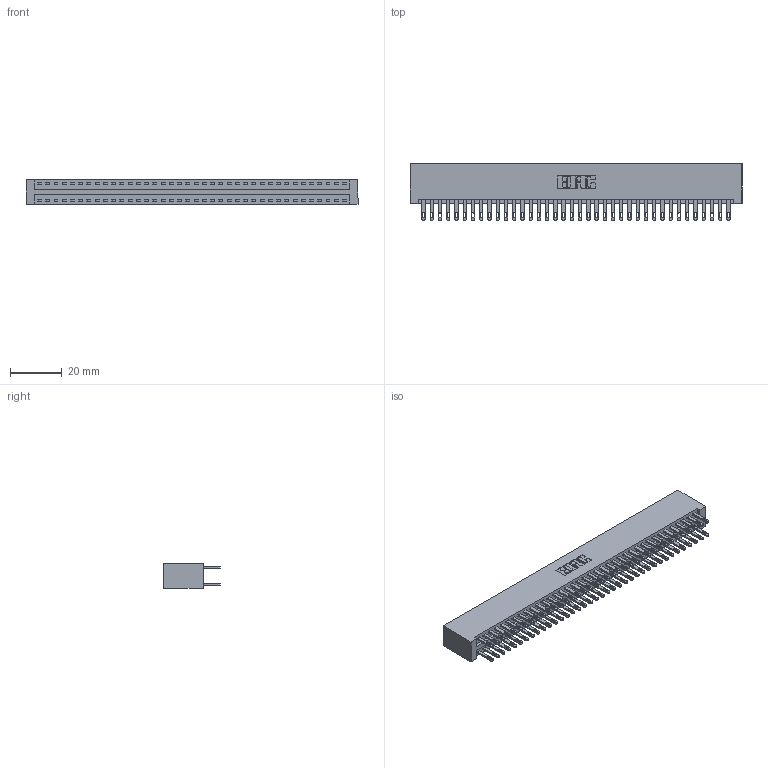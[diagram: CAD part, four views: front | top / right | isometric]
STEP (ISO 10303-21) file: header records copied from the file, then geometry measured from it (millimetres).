
FILE_DESCRIPTION (( 'STEP AP203' ), '1' );
FILE_NAME ('346-076-500-201.STEP', '2018-08-29T03:21:51', ( '' ), ( '' ), 'SwSTEP 2.0', 'SolidWorks 2016', '' );
FILE_SCHEMA (( 'CONFIG_CONTROL_DESIGN' ));
Length unit declared in the file: inch
Products named in the file (3): 346 Part_No Mounting Lugs; 345-292-001_345-293-100; 346-076-500-201
Assembly tree (77 placements, depth 2):
  346-076-500-201
    346 Part_No Mounting Lugs
    345-292-001_345-293-100  x76
Bounding box: 127.89 x 21.84 x 9.4 mm (x, y, z)
Volume: 13245.2 mm3; surface area: 19102.2 mm2
Topology: 77 solids, 77 shells, 3762 faces, 11477 edges, 7650 vertices
Faces by surface type: plane 2276, cylinder 1486
Entity records: 24991 total; most frequent: CARTESIAN_POINT 4120, ORIENTED_EDGE 4054, DIRECTION 3679, EDGE_CURVE 2027, LINE 1747, VECTOR 1747, VERTEX_POINT 1350, AXIS2_PLACEMENT_3D 966
